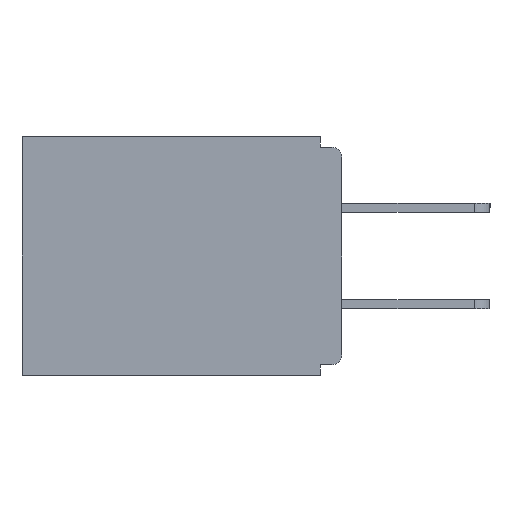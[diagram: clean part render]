
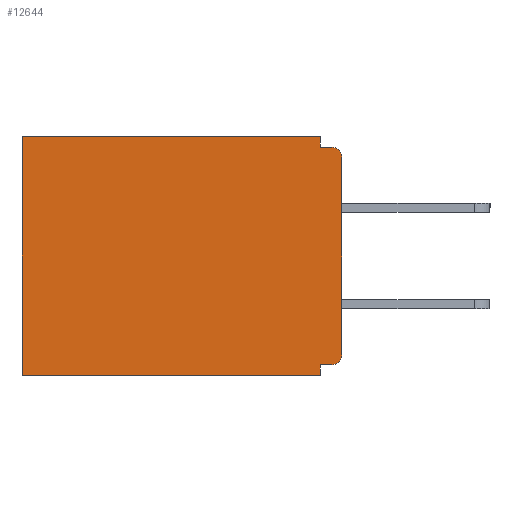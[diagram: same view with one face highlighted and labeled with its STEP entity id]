
A CAD part, left-side view. The second image highlights one B-rep face of the part: STEP entity #12644.
In plain terms, the highlighted planar face has unit normal (-1, 0, 0).
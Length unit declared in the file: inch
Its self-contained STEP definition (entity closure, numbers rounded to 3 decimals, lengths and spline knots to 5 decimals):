
#197 = LINE ( 'NONE', #10331, #7995 ) ;
#358 = PLANE ( 'NONE',  #5188 ) ;
#589 = CARTESIAN_POINT ( 'NONE',  ( 0.298, 0.031, -0.015 ) ) ;
#783 = CARTESIAN_POINT ( 'NONE',  ( 0.298, 0.031, -0.328 ) ) ;
#1096 = VECTOR ( 'NONE', #3775, 39.37008 ) ;
#1253 = EDGE_CURVE ( 'NONE', #15521, #9459, #9596, .T. ) ;
#1271 = CARTESIAN_POINT ( 'NONE',  ( 0.298, 0., 0. ) ) ;
#1550 = DIRECTION ( 'NONE',  ( 1., 0., 0. ) ) ;
#1746 = CARTESIAN_POINT ( 'NONE',  ( 0.298, 0., -0.343 ) ) ;
#2032 = AXIS2_PLACEMENT_3D ( 'NONE', #15904, #3499, #13454 ) ;
#2402 = DIRECTION ( 'NONE',  ( 0., 0., -1. ) ) ;
#2792 = ORIENTED_EDGE ( 'NONE', *, *, #12203, .T. ) ;
#3209 = CARTESIAN_POINT ( 'NONE',  ( 0.298, 0.031, -0.343 ) ) ;
#3499 = DIRECTION ( 'NONE',  ( -1., 0., 0. ) ) ;
#3502 = CARTESIAN_POINT ( 'NONE',  ( 0.298, 0., -0.328 ) ) ;
#3763 = VERTEX_POINT ( 'NONE', #14301 ) ;
#3775 = DIRECTION ( 'NONE',  ( 0., 1., 0. ) ) ;
#3805 = FACE_OUTER_BOUND ( 'NONE', #6738, .T. ) ;
#3911 = LINE ( 'NONE', #13117, #10437 ) ;
#4317 = VERTEX_POINT ( 'NONE', #15041 ) ;
#4505 = ORIENTED_EDGE ( 'NONE', *, *, #6732, .F. ) ;
#5188 = AXIS2_PLACEMENT_3D ( 'NONE', #1271, #1550, #11362 ) ;
#5324 = ORIENTED_EDGE ( 'NONE', *, *, #7968, .T. ) ;
#5434 = CARTESIAN_POINT ( 'NONE',  ( 0.298, 0.031, -0.343 ) ) ;
#5477 = VERTEX_POINT ( 'NONE', #8098 ) ;
#6620 = VECTOR ( 'NONE', #7223, 39.37008 ) ;
#6732 = EDGE_CURVE ( 'NONE', #6777, #7416, #9683, .T. ) ;
#6738 = EDGE_LOOP ( 'NONE', ( #5324, #15186, #6793, #9468, #15408, #15311, #10688, #10395, #2792, #4505 ) ) ;
#6777 = VERTEX_POINT ( 'NONE', #12338 ) ;
#6793 = ORIENTED_EDGE ( 'NONE', *, *, #11195, .F. ) ;
#6954 = DIRECTION ( 'NONE',  ( 0., 1., 0. ) ) ;
#7168 = VERTEX_POINT ( 'NONE', #10113 ) ;
#7223 = DIRECTION ( 'NONE',  ( 0., 1., 0. ) ) ;
#7360 = CIRCLE ( 'NONE', #13436, 0.015 ) ;
#7416 = VERTEX_POINT ( 'NONE', #8675 ) ;
#7949 = CARTESIAN_POINT ( 'NONE',  ( 0.298, 0., 0. ) ) ;
#7968 = EDGE_CURVE ( 'NONE', #6777, #3763, #10892, .T. ) ;
#7995 = VECTOR ( 'NONE', #11490, 39.37008 ) ;
#8098 = CARTESIAN_POINT ( 'NONE',  ( 0.298, 0.031, 0. ) ) ;
#8189 = CARTESIAN_POINT ( 'NONE',  ( 0.298, 0., 0. ) ) ;
#8226 = DIRECTION ( 'NONE',  ( 0., -1., 0. ) ) ;
#8625 = VECTOR ( 'NONE', #9070, 39.37008 ) ;
#8675 = CARTESIAN_POINT ( 'NONE',  ( 0.298, 0., -0.313 ) ) ;
#9070 = DIRECTION ( 'NONE',  ( 0., 0., -1. ) ) ;
#9459 = VERTEX_POINT ( 'NONE', #783 ) ;
#9468 = ORIENTED_EDGE ( 'NONE', *, *, #12376, .T. ) ;
#9596 = LINE ( 'NONE', #3502, #6620 ) ;
#9683 = LINE ( 'NONE', #7949, #11908 ) ;
#9725 = VECTOR ( 'NONE', #6954, 39.37008 ) ;
#10113 = CARTESIAN_POINT ( 'NONE',  ( 0.298, 0.46, 0. ) ) ;
#10331 = CARTESIAN_POINT ( 'NONE',  ( 0.298, 0.031, -0.343 ) ) ;
#10395 = ORIENTED_EDGE ( 'NONE', *, *, #1253, .F. ) ;
#10437 = VECTOR ( 'NONE', #8226, 39.37008 ) ;
#10688 = ORIENTED_EDGE ( 'NONE', *, *, #15646, .F. ) ;
#10892 = CIRCLE ( 'NONE', #2032, 0.015 ) ;
#11195 = EDGE_CURVE ( 'NONE', #5477, #13455, #197, .T. ) ;
#11362 = DIRECTION ( 'NONE',  ( 0., 0., -1. ) ) ;
#11490 = DIRECTION ( 'NONE',  ( 0., 0., -1. ) ) ;
#11685 = DIRECTION ( 'NONE',  ( 0., 0., -1. ) ) ;
#11908 = VECTOR ( 'NONE', #16225, 39.37008 ) ;
#12025 = LINE ( 'NONE', #5434, #8625 ) ;
#12132 = EDGE_CURVE ( 'NONE', #14857, #4317, #12723, .T. ) ;
#12203 = EDGE_CURVE ( 'NONE', #15521, #7416, #7360, .T. ) ;
#12293 = VECTOR ( 'NONE', #2402, 39.37008 ) ;
#12309 = LINE ( 'NONE', #8189, #9725 ) ;
#12338 = CARTESIAN_POINT ( 'NONE',  ( 0.298, 0., -0.03 ) ) ;
#12376 = EDGE_CURVE ( 'NONE', #5477, #7168, #12309, .T. ) ;
#12563 = CARTESIAN_POINT ( 'NONE',  ( 0.298, 0.015, -0.328 ) ) ;
#12644 = ADVANCED_FACE ( 'NONE', ( #3805 ), #358, .F. ) ;
#12723 = LINE ( 'NONE', #1746, #1096 ) ;
#12853 = EDGE_CURVE ( 'NONE', #7168, #4317, #13049, .T. ) ;
#13049 = LINE ( 'NONE', #14913, #12293 ) ;
#13051 = CARTESIAN_POINT ( 'NONE',  ( 0.298, 0.015, -0.313 ) ) ;
#13117 = CARTESIAN_POINT ( 'NONE',  ( 0.298, 0., -0.015 ) ) ;
#13436 = AXIS2_PLACEMENT_3D ( 'NONE', #13051, #15423, #11685 ) ;
#13454 = DIRECTION ( 'NONE',  ( 0., 0., -1. ) ) ;
#13455 = VERTEX_POINT ( 'NONE', #589 ) ;
#14301 = CARTESIAN_POINT ( 'NONE',  ( 0.298, 0.015, -0.015 ) ) ;
#14857 = VERTEX_POINT ( 'NONE', #3209 ) ;
#14913 = CARTESIAN_POINT ( 'NONE',  ( 0.298, 0.46, 0. ) ) ;
#15041 = CARTESIAN_POINT ( 'NONE',  ( 0.298, 0.46, -0.343 ) ) ;
#15186 = ORIENTED_EDGE ( 'NONE', *, *, #15816, .F. ) ;
#15311 = ORIENTED_EDGE ( 'NONE', *, *, #12132, .F. ) ;
#15408 = ORIENTED_EDGE ( 'NONE', *, *, #12853, .T. ) ;
#15423 = DIRECTION ( 'NONE',  ( -1., 0., 0. ) ) ;
#15521 = VERTEX_POINT ( 'NONE', #12563 ) ;
#15646 = EDGE_CURVE ( 'NONE', #9459, #14857, #12025, .T. ) ;
#15816 = EDGE_CURVE ( 'NONE', #13455, #3763, #3911, .T. ) ;
#15904 = CARTESIAN_POINT ( 'NONE',  ( 0.298, 0.015, -0.03 ) ) ;
#16225 = DIRECTION ( 'NONE',  ( 0., 0., -1. ) ) ;
